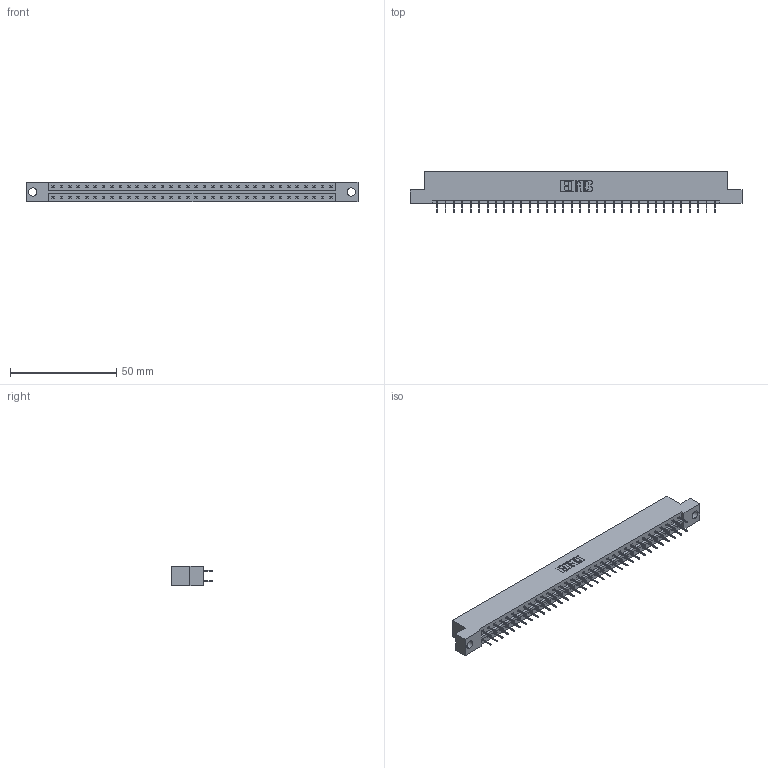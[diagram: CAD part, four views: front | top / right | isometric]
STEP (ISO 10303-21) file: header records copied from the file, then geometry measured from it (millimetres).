
FILE_DESCRIPTION (( 'STEP AP203' ), '1' );
FILE_NAME ('833-068-524-204.STEP', '2020-06-05T10:26:56', ( '' ), ( '' ), 'SwSTEP 2.0', 'SolidWorks 2020', '' );
FILE_SCHEMA (( 'CONFIG_CONTROL_DESIGN' ));
Length unit declared in the file: inch
Products named in the file (3): 345-292-001_345-293-124; 833-068-524-204; 833 Part_Flush - .156 Dia - TH
Assembly tree (69 placements, depth 2):
  833-068-524-204
    833 Part_Flush - .156 Dia - TH
    345-292-001_345-293-124  x68
Bounding box: 156.26 x 19.69 x 9.4 mm (x, y, z)
Volume: 15687.8 mm3; surface area: 17951.4 mm2
Topology: 69 solids, 69 shells, 3922 faces, 11123 edges, 7142 vertices
Faces by surface type: plane 2926, cylinder 996
Entity records: 22985 total; most frequent: CARTESIAN_POINT 3818, ORIENTED_EDGE 3754, DIRECTION 3277, EDGE_CURVE 1877, LINE 1753, VECTOR 1753, VERTEX_POINT 1246, AXIS2_PLACEMENT_3D 762
